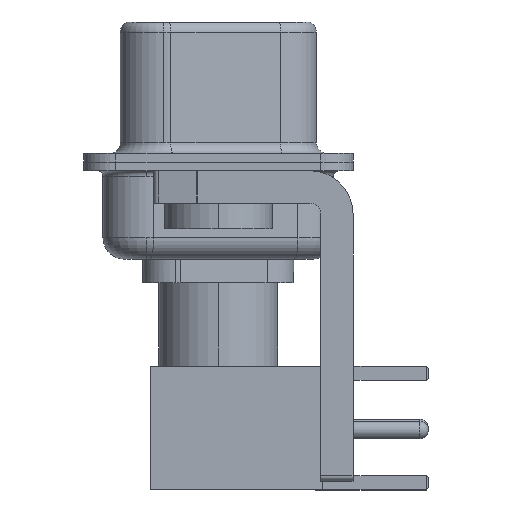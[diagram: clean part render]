
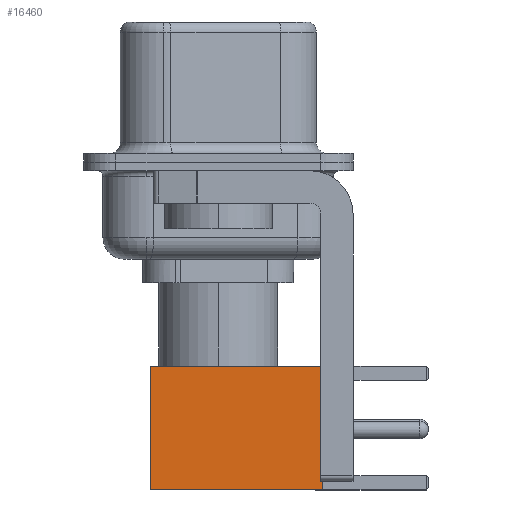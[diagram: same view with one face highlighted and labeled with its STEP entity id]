
A CAD part, left-side view. The second image highlights one B-rep face of the part: STEP entity #16460.
In plain terms, the highlighted face is planar.
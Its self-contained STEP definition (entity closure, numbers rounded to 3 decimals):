
#795 = EDGE_LOOP ( 'NONE', ( #20421, #5542, #16830, #13866 ) ) ;
#2433 = DIRECTION ( 'NONE',  ( 0., 0., 1. ) ) ;
#3461 = VERTEX_POINT ( 'NONE', #19743 ) ;
#3983 = PLANE ( 'NONE',  #11480 ) ;
#5153 = VECTOR ( 'NONE', #11340, 1000. ) ;
#5542 = ORIENTED_EDGE ( 'NONE', *, *, #10715, .T. ) ;
#6661 = CARTESIAN_POINT ( 'NONE',  ( -2.875, 2.875, 8. ) ) ;
#6859 = LINE ( 'NONE', #13305, #5153 ) ;
#6981 = LINE ( 'NONE', #7291, #20266 ) ;
#7291 = CARTESIAN_POINT ( 'NONE',  ( 2.875, 2.875, 0. ) ) ;
#8672 = LINE ( 'NONE', #14994, #14581 ) ;
#8841 = EDGE_CURVE ( 'NONE', #18558, #19387, #6981, .T. ) ;
#8868 = CARTESIAN_POINT ( 'NONE',  ( 2.875, 2.875, 0. ) ) ;
#9014 = LINE ( 'NONE', #10677, #11238 ) ;
#9355 = EDGE_CURVE ( 'NONE', #10982, #3461, #9014, .T. ) ;
#9455 = CARTESIAN_POINT ( 'NONE',  ( 2.875, 2.875, 0. ) ) ;
#10677 = CARTESIAN_POINT ( 'NONE',  ( -2.875, 2.875, 0. ) ) ;
#10715 = EDGE_CURVE ( 'NONE', #19387, #3461, #8672, .T. ) ;
#10982 = VERTEX_POINT ( 'NONE', #6661 ) ;
#11238 = VECTOR ( 'NONE', #12220, 1000. ) ;
#11340 = DIRECTION ( 'NONE',  ( -1., 0., 0. ) ) ;
#11480 = AXIS2_PLACEMENT_3D ( 'NONE', #8868, #16639, #2433 ) ;
#12220 = DIRECTION ( 'NONE',  ( 0., 0., -1. ) ) ;
#13305 = CARTESIAN_POINT ( 'NONE',  ( 0., 2.875, 8. ) ) ;
#13433 = DIRECTION ( 'NONE',  ( -1., 0., 0. ) ) ;
#13866 = ORIENTED_EDGE ( 'NONE', *, *, #16704, .F. ) ;
#14427 = CARTESIAN_POINT ( 'NONE',  ( 2.875, 2.875, 8. ) ) ;
#14581 = VECTOR ( 'NONE', #13433, 1000. ) ;
#14994 = CARTESIAN_POINT ( 'NONE',  ( 0., 2.875, 0. ) ) ;
#16460 = ADVANCED_FACE ( 'NONE', ( #18173 ), #3983, .T. ) ;
#16625 = DIRECTION ( 'NONE',  ( 0., 0., -1. ) ) ;
#16639 = DIRECTION ( 'NONE',  ( 0., 1., 0. ) ) ;
#16704 = EDGE_CURVE ( 'NONE', #18558, #10982, #6859, .T. ) ;
#16830 = ORIENTED_EDGE ( 'NONE', *, *, #9355, .F. ) ;
#18173 = FACE_OUTER_BOUND ( 'NONE', #795, .T. ) ;
#18558 = VERTEX_POINT ( 'NONE', #14427 ) ;
#19387 = VERTEX_POINT ( 'NONE', #9455 ) ;
#19743 = CARTESIAN_POINT ( 'NONE',  ( -2.875, 2.875, 0. ) ) ;
#20266 = VECTOR ( 'NONE', #16625, 1000. ) ;
#20421 = ORIENTED_EDGE ( 'NONE', *, *, #8841, .T. ) ;
